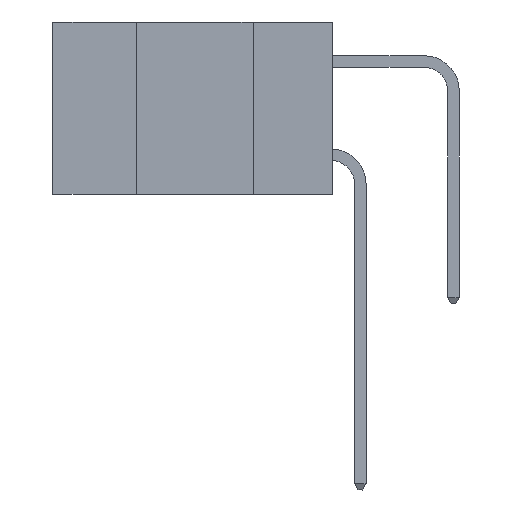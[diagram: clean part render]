
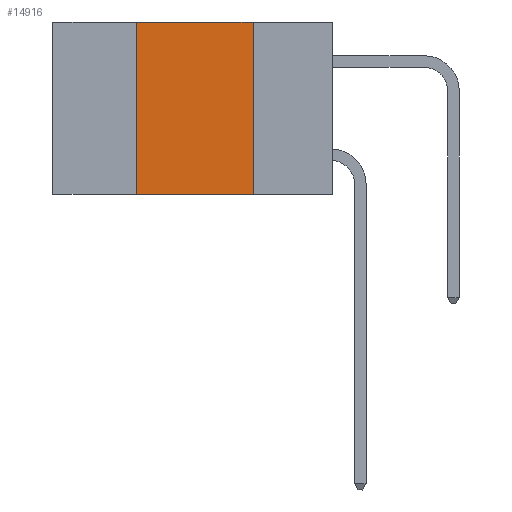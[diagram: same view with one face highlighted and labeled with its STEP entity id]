
A CAD part, left-side view. The second image highlights one B-rep face of the part: STEP entity #14916.
In plain terms, the highlighted planar face has unit normal (-1, 0, 0).
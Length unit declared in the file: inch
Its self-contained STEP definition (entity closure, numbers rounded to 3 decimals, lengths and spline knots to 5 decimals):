
#166 = VERTEX_POINT ( 'NONE', #14802 ) ;
#292 = EDGE_CURVE ( 'NONE', #11142, #14336, #9736, .T. ) ;
#389 = VECTOR ( 'NONE', #9391, 39.37008 ) ;
#575 = VERTEX_POINT ( 'NONE', #14870 ) ;
#1082 = DIRECTION ( 'NONE',  ( 0., -1., 0. ) ) ;
#1098 = PLANE ( 'NONE',  #13808 ) ;
#1889 = ORIENTED_EDGE ( 'NONE', *, *, #6326, .F. ) ;
#2124 = FACE_OUTER_BOUND ( 'NONE', #8523, .T. ) ;
#2179 = LINE ( 'NONE', #10707, #14253 ) ;
#4555 = CARTESIAN_POINT ( 'NONE',  ( 0., 0.6, 0. ) ) ;
#4606 = DIRECTION ( 'NONE',  ( 0., 0., -1. ) ) ;
#4621 = CARTESIAN_POINT ( 'NONE',  ( 0., 0.42, 0. ) ) ;
#4764 = EDGE_CURVE ( 'NONE', #11142, #575, #14275, .T. ) ;
#4905 = LINE ( 'NONE', #12778, #7991 ) ;
#5651 = CARTESIAN_POINT ( 'NONE',  ( 0., 0.42, 0. ) ) ;
#6073 = DIRECTION ( 'NONE',  ( 0., -1., 0. ) ) ;
#6326 = EDGE_CURVE ( 'NONE', #166, #575, #2179, .T. ) ;
#6519 = CARTESIAN_POINT ( 'NONE',  ( 0., 0.42, -0.37 ) ) ;
#7991 = VECTOR ( 'NONE', #1082, 39.37008 ) ;
#8523 = EDGE_LOOP ( 'NONE', ( #1889, #13802, #13227, #9024 ) ) ;
#9024 = ORIENTED_EDGE ( 'NONE', *, *, #4764, .T. ) ;
#9391 = DIRECTION ( 'NONE',  ( 0., 0., 1. ) ) ;
#9736 = LINE ( 'NONE', #5651, #389 ) ;
#10707 = CARTESIAN_POINT ( 'NONE',  ( 0., 0.17, 0. ) ) ;
#11142 = VERTEX_POINT ( 'NONE', #6519 ) ;
#11553 = VECTOR ( 'NONE', #6073, 39.37008 ) ;
#11644 = DIRECTION ( 'NONE',  ( 1., 0., 0. ) ) ;
#12543 = CARTESIAN_POINT ( 'NONE',  ( 0., 0.6, -0.37 ) ) ;
#12778 = CARTESIAN_POINT ( 'NONE',  ( 0., 0.6, 0. ) ) ;
#13227 = ORIENTED_EDGE ( 'NONE', *, *, #292, .F. ) ;
#13652 = EDGE_CURVE ( 'NONE', #14336, #166, #4905, .T. ) ;
#13802 = ORIENTED_EDGE ( 'NONE', *, *, #13652, .F. ) ;
#13808 = AXIS2_PLACEMENT_3D ( 'NONE', #4555, #11644, #4606 ) ;
#14253 = VECTOR ( 'NONE', #14941, 39.37008 ) ;
#14275 = LINE ( 'NONE', #12543, #11553 ) ;
#14336 = VERTEX_POINT ( 'NONE', #4621 ) ;
#14802 = CARTESIAN_POINT ( 'NONE',  ( 0., 0.17, 0. ) ) ;
#14870 = CARTESIAN_POINT ( 'NONE',  ( 0., 0.17, -0.37 ) ) ;
#14916 = ADVANCED_FACE ( 'NONE', ( #2124 ), #1098, .F. ) ;
#14941 = DIRECTION ( 'NONE',  ( 0., 0., -1. ) ) ;
